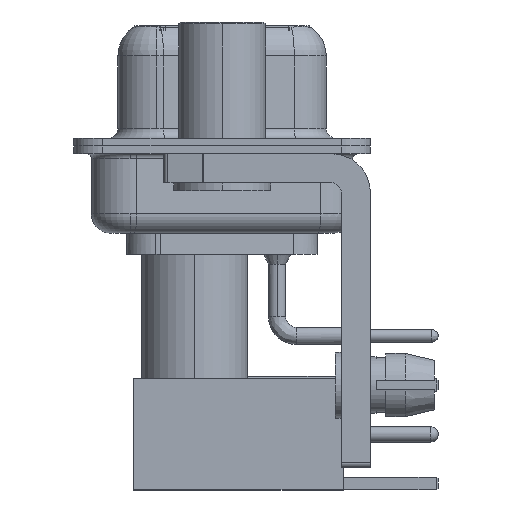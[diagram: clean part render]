
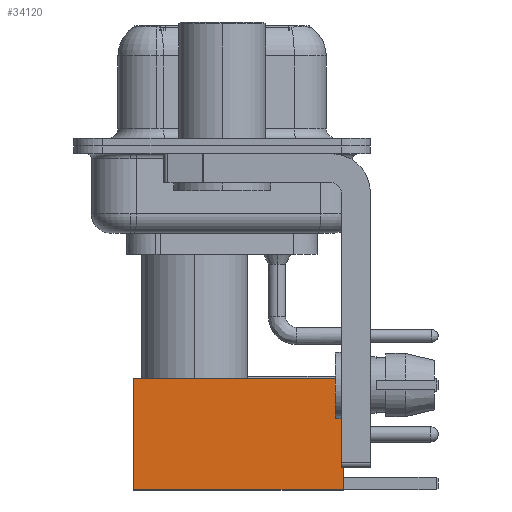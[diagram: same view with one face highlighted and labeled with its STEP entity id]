
A CAD part, left-side view. The second image highlights one B-rep face of the part: STEP entity #34120.
In plain terms, the highlighted face is planar.
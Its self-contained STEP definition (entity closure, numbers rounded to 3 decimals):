
#697 = DIRECTION ( 'NONE',  ( 0., 0., -1. ) ) ;
#1251 = DIRECTION ( 'NONE',  ( 0., 0., 1. ) ) ;
#4271 = DIRECTION ( 'NONE',  ( 0., 1., 0. ) ) ;
#4785 = LINE ( 'NONE', #7058, #23471 ) ;
#5258 = VECTOR ( 'NONE', #10788, 1000. ) ;
#6100 = CARTESIAN_POINT ( 'NONE',  ( 2.875, 2.875, 0. ) ) ;
#6554 = CARTESIAN_POINT ( 'NONE',  ( 2.875, 2.875, 0. ) ) ;
#7058 = CARTESIAN_POINT ( 'NONE',  ( 0., 2.875, 10.82 ) ) ;
#8270 = LINE ( 'NONE', #29500, #21162 ) ;
#9073 = CARTESIAN_POINT ( 'NONE',  ( -2.875, 2.875, 0. ) ) ;
#10090 = AXIS2_PLACEMENT_3D ( 'NONE', #6554, #4271, #1251 ) ;
#10103 = ORIENTED_EDGE ( 'NONE', *, *, #28601, .F. ) ;
#10788 = DIRECTION ( 'NONE',  ( -1., 0., 0. ) ) ;
#11241 = EDGE_CURVE ( 'NONE', #32350, #30902, #31645, .T. ) ;
#11534 = ORIENTED_EDGE ( 'NONE', *, *, #30369, .T. ) ;
#12647 = ORIENTED_EDGE ( 'NONE', *, *, #34799, .F. ) ;
#12842 = VERTEX_POINT ( 'NONE', #13252 ) ;
#13252 = CARTESIAN_POINT ( 'NONE',  ( -2.875, 2.875, 10.82 ) ) ;
#15731 = LINE ( 'NONE', #29599, #30871 ) ;
#17796 = VERTEX_POINT ( 'NONE', #21013 ) ;
#17821 = DIRECTION ( 'NONE',  ( 0., 0., -1. ) ) ;
#21013 = CARTESIAN_POINT ( 'NONE',  ( 2.875, 2.875, 10.82 ) ) ;
#21162 = VECTOR ( 'NONE', #697, 1000. ) ;
#23471 = VECTOR ( 'NONE', #30196, 1000. ) ;
#23652 = ORIENTED_EDGE ( 'NONE', *, *, #11241, .T. ) ;
#26665 = PLANE ( 'NONE',  #10090 ) ;
#28601 = EDGE_CURVE ( 'NONE', #12842, #30902, #8270, .T. ) ;
#29500 = CARTESIAN_POINT ( 'NONE',  ( -2.875, 2.875, 0. ) ) ;
#29599 = CARTESIAN_POINT ( 'NONE',  ( 2.875, 2.875, 0. ) ) ;
#30053 = FACE_OUTER_BOUND ( 'NONE', #34683, .T. ) ;
#30196 = DIRECTION ( 'NONE',  ( -1., 0., 0. ) ) ;
#30369 = EDGE_CURVE ( 'NONE', #17796, #32350, #15731, .T. ) ;
#30871 = VECTOR ( 'NONE', #17821, 1000. ) ;
#30902 = VERTEX_POINT ( 'NONE', #9073 ) ;
#31448 = CARTESIAN_POINT ( 'NONE',  ( 0., 2.875, 0. ) ) ;
#31645 = LINE ( 'NONE', #31448, #5258 ) ;
#32350 = VERTEX_POINT ( 'NONE', #6100 ) ;
#34120 = ADVANCED_FACE ( 'NONE', ( #30053 ), #26665, .T. ) ;
#34683 = EDGE_LOOP ( 'NONE', ( #11534, #23652, #10103, #12647 ) ) ;
#34799 = EDGE_CURVE ( 'NONE', #17796, #12842, #4785, .T. ) ;
